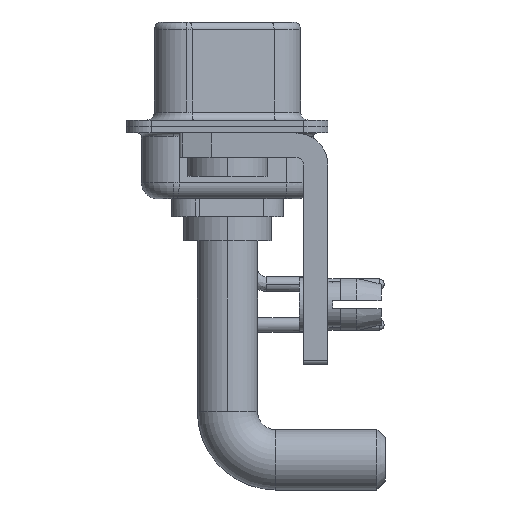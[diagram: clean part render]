
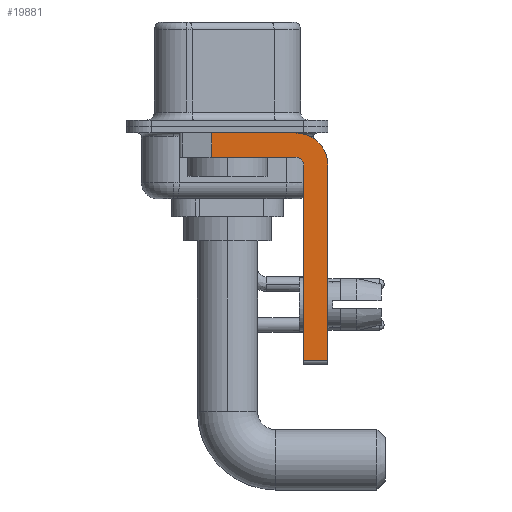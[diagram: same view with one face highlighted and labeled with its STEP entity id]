
A CAD part, left-side view. The second image highlights one B-rep face of the part: STEP entity #19881.
In plain terms, the highlighted planar face has unit normal (-1, 0, 0).
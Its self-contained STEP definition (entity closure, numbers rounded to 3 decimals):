
#636 = VERTEX_POINT ( 'NONE', #20897 ) ;
#1046 = VECTOR ( 'NONE', #2366, 1000. ) ;
#1434 = DIRECTION ( 'NONE',  ( 1., 0., 0. ) ) ;
#2366 = DIRECTION ( 'NONE',  ( 0., -1., 0. ) ) ;
#3073 = LINE ( 'NONE', #15677, #16458 ) ;
#3176 = CARTESIAN_POINT ( 'NONE',  ( -2.9, -6.25, -14.55 ) ) ;
#3221 = DIRECTION ( 'NONE',  ( 0., 1., 0. ) ) ;
#4091 = CARTESIAN_POINT ( 'NONE',  ( -2.9, 0.978, -1.9 ) ) ;
#4107 = LINE ( 'NONE', #24761, #18393 ) ;
#4353 = ORIENTED_EDGE ( 'NONE', *, *, #13420, .F. ) ;
#4719 = CARTESIAN_POINT ( 'NONE',  ( -2.9, -4.25, -0.4 ) ) ;
#5820 = CARTESIAN_POINT ( 'NONE',  ( -2.9, -4.75, -14.8 ) ) ;
#6127 = VECTOR ( 'NONE', #3221, 1000. ) ;
#6140 = ORIENTED_EDGE ( 'NONE', *, *, #24510, .T. ) ;
#6192 = ORIENTED_EDGE ( 'NONE', *, *, #25952, .F. ) ;
#6523 = ORIENTED_EDGE ( 'NONE', *, *, #24182, .F. ) ;
#6538 = DIRECTION ( 'NONE',  ( 0., 0., -1. ) ) ;
#7016 = AXIS2_PLACEMENT_3D ( 'NONE', #14493, #10524, #16270 ) ;
#7291 = VERTEX_POINT ( 'NONE', #18107 ) ;
#7458 = EDGE_CURVE ( 'NONE', #26288, #10765, #4107, .T. ) ;
#7871 = LINE ( 'NONE', #16368, #9105 ) ;
#8597 = PLANE ( 'NONE',  #21227 ) ;
#8933 = LINE ( 'NONE', #11006, #1046 ) ;
#9105 = VECTOR ( 'NONE', #22663, 1000. ) ;
#9172 = EDGE_CURVE ( 'NONE', #7291, #15273, #23216, .T. ) ;
#10218 = DIRECTION ( 'NONE',  ( 0., 0., 1. ) ) ;
#10352 = CIRCLE ( 'NONE', #13411, 2. ) ;
#10524 = DIRECTION ( 'NONE',  ( -1., 0., 0. ) ) ;
#10765 = VERTEX_POINT ( 'NONE', #3176 ) ;
#11006 = CARTESIAN_POINT ( 'NONE',  ( -2.9, 3., -0.4 ) ) ;
#11998 = EDGE_CURVE ( 'NONE', #636, #16170, #8933, .T. ) ;
#13051 = CARTESIAN_POINT ( 'NONE',  ( -2.9, -6.25, -2.4 ) ) ;
#13329 = EDGE_LOOP ( 'NONE', ( #23722, #24826, #4353, #17972, #6523, #6140, #25712, #6192 ) ) ;
#13411 = AXIS2_PLACEMENT_3D ( 'NONE', #24813, #1434, #20455 ) ;
#13420 = EDGE_CURVE ( 'NONE', #15273, #18579, #21590, .T. ) ;
#14189 = LINE ( 'NONE', #5820, #20042 ) ;
#14493 = CARTESIAN_POINT ( 'NONE',  ( -2.9, -4.25, -2.4 ) ) ;
#14775 = CARTESIAN_POINT ( 'NONE',  ( -2.9, -4.25, -2.4 ) ) ;
#15273 = VERTEX_POINT ( 'NONE', #17940 ) ;
#15677 = CARTESIAN_POINT ( 'NONE',  ( -2.9, -4.25, -14.55 ) ) ;
#16170 = VERTEX_POINT ( 'NONE', #4719 ) ;
#16270 = DIRECTION ( 'NONE',  ( 0., 0., 1. ) ) ;
#16368 = CARTESIAN_POINT ( 'NONE',  ( -2.9, 0.978, -1.9 ) ) ;
#16458 = VECTOR ( 'NONE', #24023, 1000. ) ;
#16711 = CARTESIAN_POINT ( 'NONE',  ( -2.9, -4.75, -14.55 ) ) ;
#16964 = DIRECTION ( 'NONE',  ( 1., 0., 0. ) ) ;
#17940 = CARTESIAN_POINT ( 'NONE',  ( -2.9, -4.25, -1.9 ) ) ;
#17972 = ORIENTED_EDGE ( 'NONE', *, *, #9172, .F. ) ;
#18107 = CARTESIAN_POINT ( 'NONE',  ( -2.9, -4.75, -2.4 ) ) ;
#18393 = VECTOR ( 'NONE', #20815, 1000. ) ;
#18579 = VERTEX_POINT ( 'NONE', #4091 ) ;
#19881 = ADVANCED_FACE ( 'NONE', ( #20939 ), #8597, .F. ) ;
#20042 = VECTOR ( 'NONE', #10218, 1000. ) ;
#20455 = DIRECTION ( 'NONE',  ( 0., 0., -1. ) ) ;
#20815 = DIRECTION ( 'NONE',  ( 0., 0., -1. ) ) ;
#20897 = CARTESIAN_POINT ( 'NONE',  ( -2.9, 0.978, -0.4 ) ) ;
#20939 = FACE_OUTER_BOUND ( 'NONE', #13329, .T. ) ;
#21227 = AXIS2_PLACEMENT_3D ( 'NONE', #14775, #16964, #6538 ) ;
#21590 = LINE ( 'NONE', #23897, #6127 ) ;
#22100 = VERTEX_POINT ( 'NONE', #16711 ) ;
#22663 = DIRECTION ( 'NONE',  ( 0., 0., -1. ) ) ;
#23216 = CIRCLE ( 'NONE', #7016, 0.5 ) ;
#23722 = ORIENTED_EDGE ( 'NONE', *, *, #11998, .F. ) ;
#23897 = CARTESIAN_POINT ( 'NONE',  ( -2.9, -4.25, -1.9 ) ) ;
#24023 = DIRECTION ( 'NONE',  ( 0., -1., 0. ) ) ;
#24152 = EDGE_CURVE ( 'NONE', #636, #18579, #7871, .T. ) ;
#24182 = EDGE_CURVE ( 'NONE', #22100, #7291, #14189, .T. ) ;
#24510 = EDGE_CURVE ( 'NONE', #22100, #10765, #3073, .T. ) ;
#24761 = CARTESIAN_POINT ( 'NONE',  ( -2.9, -6.25, -2.4 ) ) ;
#24813 = CARTESIAN_POINT ( 'NONE',  ( -2.9, -4.25, -2.4 ) ) ;
#24826 = ORIENTED_EDGE ( 'NONE', *, *, #24152, .T. ) ;
#25712 = ORIENTED_EDGE ( 'NONE', *, *, #7458, .F. ) ;
#25952 = EDGE_CURVE ( 'NONE', #16170, #26288, #10352, .T. ) ;
#26288 = VERTEX_POINT ( 'NONE', #13051 ) ;
